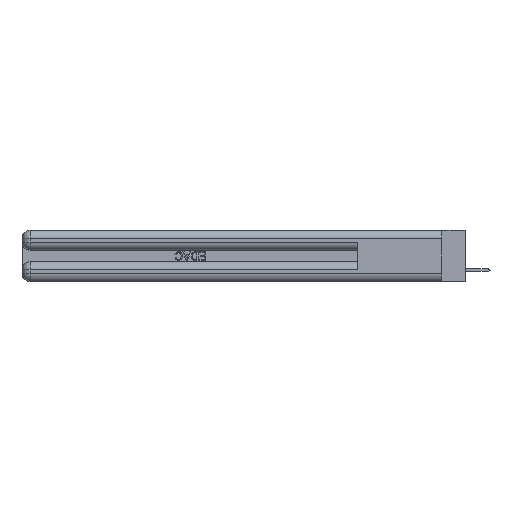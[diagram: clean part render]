
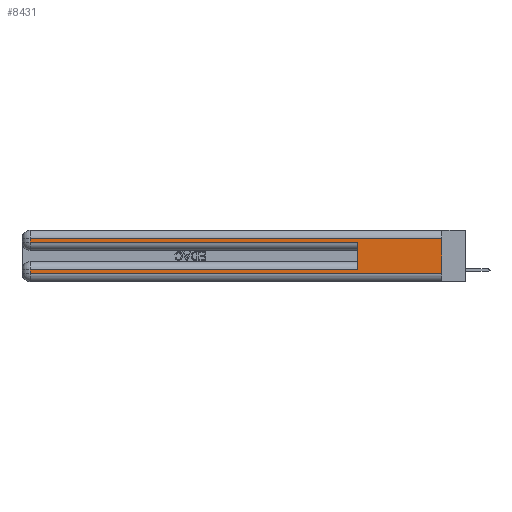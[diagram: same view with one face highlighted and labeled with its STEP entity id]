
A CAD part, left-side view. The second image highlights one B-rep face of the part: STEP entity #8431.
In plain terms, the highlighted planar face has unit normal (-1, 0, 0).
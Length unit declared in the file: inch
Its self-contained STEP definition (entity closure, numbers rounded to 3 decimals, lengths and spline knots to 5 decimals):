
#1242 = LINE ( 'NONE', #7002, #32272 ) ;
#1768 = EDGE_CURVE ( 'NONE', #18850, #13275, #28719, .T. ) ;
#1784 = CARTESIAN_POINT ( 'NONE',  ( 0., 0.6, 0.085 ) ) ;
#2180 = ORIENTED_EDGE ( 'NONE', *, *, #13024, .T. ) ;
#2823 = ORIENTED_EDGE ( 'NONE', *, *, #35709, .T. ) ;
#4217 = CARTESIAN_POINT ( 'NONE',  ( 0., 2.94, 0.31 ) ) ;
#4254 = DIRECTION ( 'NONE',  ( 0., 0., -1. ) ) ;
#5770 = CARTESIAN_POINT ( 'NONE',  ( 0., 0., 0.085 ) ) ;
#5962 = VECTOR ( 'NONE', #28431, 39.37008 ) ;
#6630 = EDGE_CURVE ( 'NONE', #17532, #31672, #18906, .T. ) ;
#6638 = ORIENTED_EDGE ( 'NONE', *, *, #21163, .F. ) ;
#7002 = CARTESIAN_POINT ( 'NONE',  ( 0., 2.94, 0.37 ) ) ;
#7142 = VECTOR ( 'NONE', #15729, 39.37008 ) ;
#7429 = CARTESIAN_POINT ( 'NONE',  ( 0., 0., 0.06 ) ) ;
#7760 = VERTEX_POINT ( 'NONE', #33285 ) ;
#7973 = VERTEX_POINT ( 'NONE', #11004 ) ;
#8082 = VECTOR ( 'NONE', #22722, 39.37008 ) ;
#8358 = DIRECTION ( 'NONE',  ( 0., 0., -1. ) ) ;
#8431 = ADVANCED_FACE ( 'NONE', ( #36597 ), #24386, .F. ) ;
#8498 = CARTESIAN_POINT ( 'NONE',  ( 0., 0., 0.06 ) ) ;
#9080 = ORIENTED_EDGE ( 'NONE', *, *, #6630, .T. ) ;
#10968 = CARTESIAN_POINT ( 'NONE',  ( 0., 2.94, 0.37 ) ) ;
#11004 = CARTESIAN_POINT ( 'NONE',  ( 0., 2.94, 0.085 ) ) ;
#12224 = LINE ( 'NONE', #10968, #35641 ) ;
#13024 = EDGE_CURVE ( 'NONE', #7973, #18850, #1242, .T. ) ;
#13275 = VERTEX_POINT ( 'NONE', #7429 ) ;
#15344 = CARTESIAN_POINT ( 'NONE',  ( 0., 0., 0.37 ) ) ;
#15729 = DIRECTION ( 'NONE',  ( 0., -1., 0. ) ) ;
#16573 = VECTOR ( 'NONE', #36315, 39.37008 ) ;
#17532 = VERTEX_POINT ( 'NONE', #35228 ) ;
#17620 = DIRECTION ( 'NONE',  ( 0., 0., -1. ) ) ;
#17703 = AXIS2_PLACEMENT_3D ( 'NONE', #33460, #21502, #4254 ) ;
#17821 = VECTOR ( 'NONE', #18012, 39.37008 ) ;
#18012 = DIRECTION ( 'NONE',  ( 0., 1., 0. ) ) ;
#18850 = VERTEX_POINT ( 'NONE', #19284 ) ;
#18906 = LINE ( 'NONE', #37419, #8082 ) ;
#19284 = CARTESIAN_POINT ( 'NONE',  ( 0., 2.94, 0.06 ) ) ;
#19385 = LINE ( 'NONE', #30420, #33925 ) ;
#20187 = EDGE_CURVE ( 'NONE', #23864, #7973, #37064, .T. ) ;
#21163 = EDGE_CURVE ( 'NONE', #23864, #31672, #23349, .T. ) ;
#21502 = DIRECTION ( 'NONE',  ( 1., 0., 0. ) ) ;
#22722 = DIRECTION ( 'NONE',  ( 0., -1., 0. ) ) ;
#23349 = LINE ( 'NONE', #31211, #5962 ) ;
#23864 = VERTEX_POINT ( 'NONE', #1784 ) ;
#24051 = LINE ( 'NONE', #15344, #16573 ) ;
#24386 = PLANE ( 'NONE',  #17703 ) ;
#24867 = ORIENTED_EDGE ( 'NONE', *, *, #20187, .T. ) ;
#27663 = DIRECTION ( 'NONE',  ( 0., 1., 0. ) ) ;
#27853 = EDGE_CURVE ( 'NONE', #7760, #13275, #24051, .T. ) ;
#28431 = DIRECTION ( 'NONE',  ( 0., 0., 1. ) ) ;
#28482 = ORIENTED_EDGE ( 'NONE', *, *, #32027, .T. ) ;
#28719 = LINE ( 'NONE', #8498, #7142 ) ;
#29395 = CARTESIAN_POINT ( 'NONE',  ( 0., 0.6, 0.285 ) ) ;
#30420 = CARTESIAN_POINT ( 'NONE',  ( 0., 0., 0.31 ) ) ;
#31211 = CARTESIAN_POINT ( 'NONE',  ( 0., 0.6, 0.145 ) ) ;
#31672 = VERTEX_POINT ( 'NONE', #29395 ) ;
#32027 = EDGE_CURVE ( 'NONE', #7760, #38362, #19385, .T. ) ;
#32272 = VECTOR ( 'NONE', #17620, 39.37008 ) ;
#33285 = CARTESIAN_POINT ( 'NONE',  ( 0., 0., 0.31 ) ) ;
#33338 = ORIENTED_EDGE ( 'NONE', *, *, #27853, .F. ) ;
#33460 = CARTESIAN_POINT ( 'NONE',  ( 0., 0., 0.37 ) ) ;
#33925 = VECTOR ( 'NONE', #27663, 39.37008 ) ;
#35228 = CARTESIAN_POINT ( 'NONE',  ( 0., 2.94, 0.285 ) ) ;
#35641 = VECTOR ( 'NONE', #8358, 39.37008 ) ;
#35709 = EDGE_CURVE ( 'NONE', #38362, #17532, #12224, .T. ) ;
#36315 = DIRECTION ( 'NONE',  ( 0., 0., -1. ) ) ;
#36425 = ORIENTED_EDGE ( 'NONE', *, *, #1768, .T. ) ;
#36597 = FACE_OUTER_BOUND ( 'NONE', #37510, .T. ) ;
#37064 = LINE ( 'NONE', #5770, #17821 ) ;
#37419 = CARTESIAN_POINT ( 'NONE',  ( 0., 0., 0.285 ) ) ;
#37510 = EDGE_LOOP ( 'NONE', ( #33338, #28482, #2823, #9080, #6638, #24867, #2180, #36425 ) ) ;
#38362 = VERTEX_POINT ( 'NONE', #4217 ) ;
